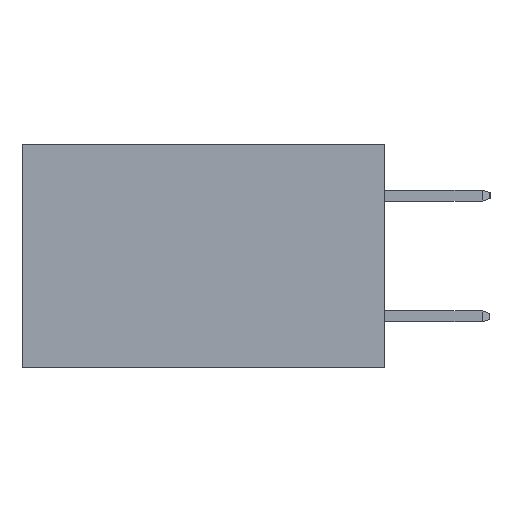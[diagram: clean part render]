
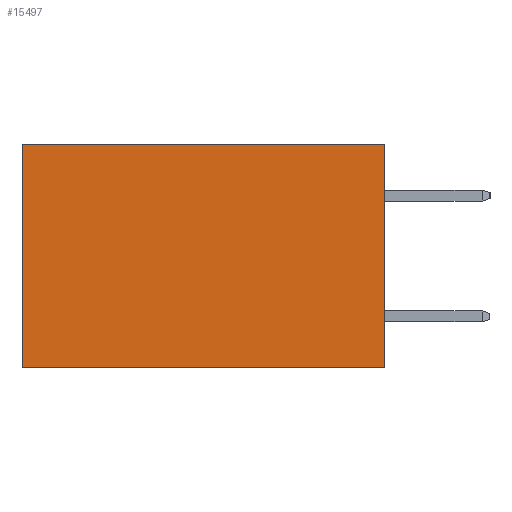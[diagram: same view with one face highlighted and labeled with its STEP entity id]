
A CAD part, left-side view. The second image highlights one B-rep face of the part: STEP entity #15497.
In plain terms, the highlighted planar face has unit normal (-1, 0, 0).
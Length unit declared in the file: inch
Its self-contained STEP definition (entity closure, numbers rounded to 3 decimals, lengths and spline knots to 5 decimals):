
#1075 = LINE ( 'NONE', #13759, #11963 ) ;
#1554 = CARTESIAN_POINT ( 'NONE',  ( 0.298, 0., 0. ) ) ;
#2244 = ORIENTED_EDGE ( 'NONE', *, *, #17680, .T. ) ;
#2848 = VERTEX_POINT ( 'NONE', #15140 ) ;
#3045 = DIRECTION ( 'NONE',  ( 0., 0., -1. ) ) ;
#5270 = ORIENTED_EDGE ( 'NONE', *, *, #12633, .T. ) ;
#5364 = EDGE_CURVE ( 'NONE', #2848, #10349, #17957, .T. ) ;
#6936 = LINE ( 'NONE', #8850, #10852 ) ;
#7514 = LINE ( 'NONE', #16434, #18439 ) ;
#8134 = AXIS2_PLACEMENT_3D ( 'NONE', #1554, #11901, #3045 ) ;
#8348 = DIRECTION ( 'NONE',  ( 0., 0., -1. ) ) ;
#8850 = CARTESIAN_POINT ( 'NONE',  ( 0.298, 0., 0. ) ) ;
#8955 = PLANE ( 'NONE',  #8134 ) ;
#9009 = DIRECTION ( 'NONE',  ( 0., 1., 0. ) ) ;
#9264 = DIRECTION ( 'NONE',  ( 0., 0., -1. ) ) ;
#10325 = CARTESIAN_POINT ( 'NONE',  ( 0.298, 0.6, 0. ) ) ;
#10349 = VERTEX_POINT ( 'NONE', #13897 ) ;
#10439 = VECTOR ( 'NONE', #9009, 39.37008 ) ;
#10852 = VECTOR ( 'NONE', #8348, 39.37008 ) ;
#11620 = FACE_OUTER_BOUND ( 'NONE', #15809, .T. ) ;
#11834 = EDGE_CURVE ( 'NONE', #14182, #2848, #6936, .T. ) ;
#11901 = DIRECTION ( 'NONE',  ( 1., 0., 0. ) ) ;
#11963 = VECTOR ( 'NONE', #17946, 39.37008 ) ;
#12617 = ORIENTED_EDGE ( 'NONE', *, *, #11834, .F. ) ;
#12633 = EDGE_CURVE ( 'NONE', #14182, #13024, #1075, .T. ) ;
#13024 = VERTEX_POINT ( 'NONE', #10325 ) ;
#13759 = CARTESIAN_POINT ( 'NONE',  ( 0.298, 0., 0. ) ) ;
#13806 = ORIENTED_EDGE ( 'NONE', *, *, #5364, .F. ) ;
#13897 = CARTESIAN_POINT ( 'NONE',  ( 0.298, 0.6, -0.37 ) ) ;
#14182 = VERTEX_POINT ( 'NONE', #15829 ) ;
#15140 = CARTESIAN_POINT ( 'NONE',  ( 0.298, 0., -0.37 ) ) ;
#15497 = ADVANCED_FACE ( 'NONE', ( #11620 ), #8955, .F. ) ;
#15809 = EDGE_LOOP ( 'NONE', ( #2244, #13806, #12617, #5270 ) ) ;
#15829 = CARTESIAN_POINT ( 'NONE',  ( 0.298, 0., 0. ) ) ;
#16185 = CARTESIAN_POINT ( 'NONE',  ( 0.298, 0., -0.37 ) ) ;
#16434 = CARTESIAN_POINT ( 'NONE',  ( 0.298, 0.6, 0. ) ) ;
#17680 = EDGE_CURVE ( 'NONE', #13024, #10349, #7514, .T. ) ;
#17946 = DIRECTION ( 'NONE',  ( 0., 1., 0. ) ) ;
#17957 = LINE ( 'NONE', #16185, #10439 ) ;
#18439 = VECTOR ( 'NONE', #9264, 39.37008 ) ;
